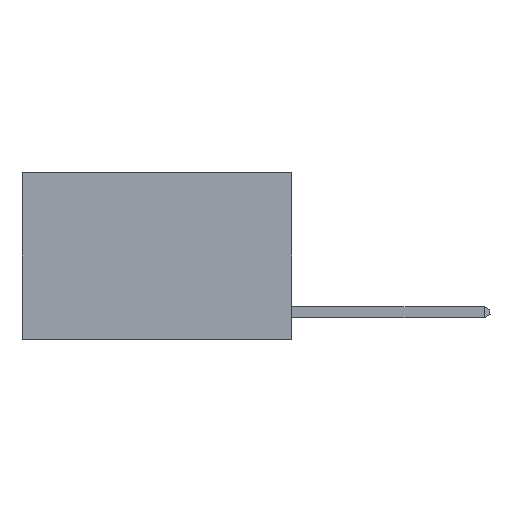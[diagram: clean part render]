
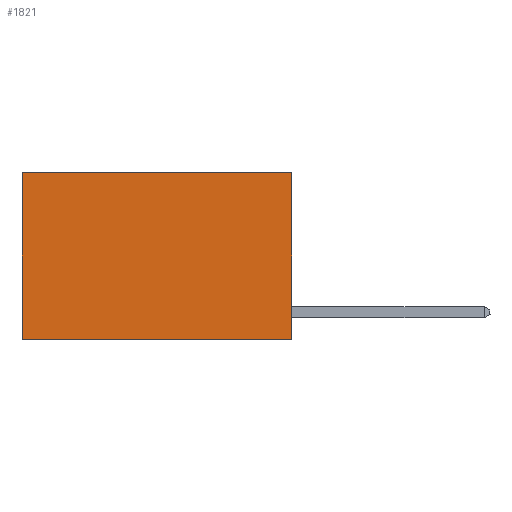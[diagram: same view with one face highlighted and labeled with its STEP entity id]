
A CAD part, left-side view. The second image highlights one B-rep face of the part: STEP entity #1821.
In plain terms, the highlighted planar face has unit normal (-1, 0, 0).
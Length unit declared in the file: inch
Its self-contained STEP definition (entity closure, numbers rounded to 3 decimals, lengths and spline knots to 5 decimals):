
#496 = CARTESIAN_POINT ( 'NONE',  ( 0.2625, 0.6, 0. ) ) ;
#526 = DIRECTION ( 'NONE',  ( 0., 1., 0. ) ) ;
#580 = DIRECTION ( 'NONE',  ( 0., 0., -1. ) ) ;
#645 = DIRECTION ( 'NONE',  ( 0., 1., 0. ) ) ;
#1623 = PLANE ( 'NONE',  #5077 ) ;
#1693 = EDGE_CURVE ( 'NONE', #7721, #3807, #6893, .T. ) ;
#1821 = ADVANCED_FACE ( 'NONE', ( #12013 ), #1623, .F. ) ;
#1914 = VERTEX_POINT ( 'NONE', #4584 ) ;
#2919 = CARTESIAN_POINT ( 'NONE',  ( 0.2625, 0.6, -0.37 ) ) ;
#3544 = DIRECTION ( 'NONE',  ( 1., 0., 0. ) ) ;
#3600 = CARTESIAN_POINT ( 'NONE',  ( 0.2625, 0., 0. ) ) ;
#3807 = VERTEX_POINT ( 'NONE', #2919 ) ;
#3902 = EDGE_LOOP ( 'NONE', ( #7966, #11167, #8921, #7482 ) ) ;
#3921 = VERTEX_POINT ( 'NONE', #11819 ) ;
#4456 = VECTOR ( 'NONE', #645, 39.37008 ) ;
#4525 = LINE ( 'NONE', #6265, #4456 ) ;
#4584 = CARTESIAN_POINT ( 'NONE',  ( 0.2625, 0., -0.37 ) ) ;
#5077 = AXIS2_PLACEMENT_3D ( 'NONE', #3600, #3544, #10201 ) ;
#5203 = LINE ( 'NONE', #8236, #6264 ) ;
#5248 = EDGE_CURVE ( 'NONE', #3921, #1914, #5203, .T. ) ;
#5281 = LINE ( 'NONE', #5341, #9838 ) ;
#5286 = VECTOR ( 'NONE', #5961, 39.37008 ) ;
#5341 = CARTESIAN_POINT ( 'NONE',  ( 0.2625, 0., 0. ) ) ;
#5961 = DIRECTION ( 'NONE',  ( 0., 0., -1. ) ) ;
#6264 = VECTOR ( 'NONE', #580, 39.37008 ) ;
#6265 = CARTESIAN_POINT ( 'NONE',  ( 0.2625, 0., -0.37 ) ) ;
#6893 = LINE ( 'NONE', #7957, #5286 ) ;
#7482 = ORIENTED_EDGE ( 'NONE', *, *, #12034, .T. ) ;
#7721 = VERTEX_POINT ( 'NONE', #496 ) ;
#7957 = CARTESIAN_POINT ( 'NONE',  ( 0.2625, 0.6, 0. ) ) ;
#7966 = ORIENTED_EDGE ( 'NONE', *, *, #1693, .T. ) ;
#8236 = CARTESIAN_POINT ( 'NONE',  ( 0.2625, 0., 0. ) ) ;
#8649 = EDGE_CURVE ( 'NONE', #1914, #3807, #4525, .T. ) ;
#8921 = ORIENTED_EDGE ( 'NONE', *, *, #5248, .F. ) ;
#9838 = VECTOR ( 'NONE', #526, 39.37008 ) ;
#10201 = DIRECTION ( 'NONE',  ( 0., 0., -1. ) ) ;
#11167 = ORIENTED_EDGE ( 'NONE', *, *, #8649, .F. ) ;
#11819 = CARTESIAN_POINT ( 'NONE',  ( 0.2625, 0., 0. ) ) ;
#12013 = FACE_OUTER_BOUND ( 'NONE', #3902, .T. ) ;
#12034 = EDGE_CURVE ( 'NONE', #3921, #7721, #5281, .T. ) ;
